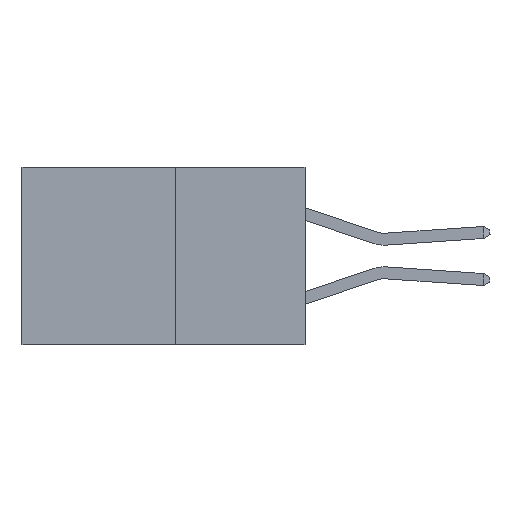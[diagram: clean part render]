
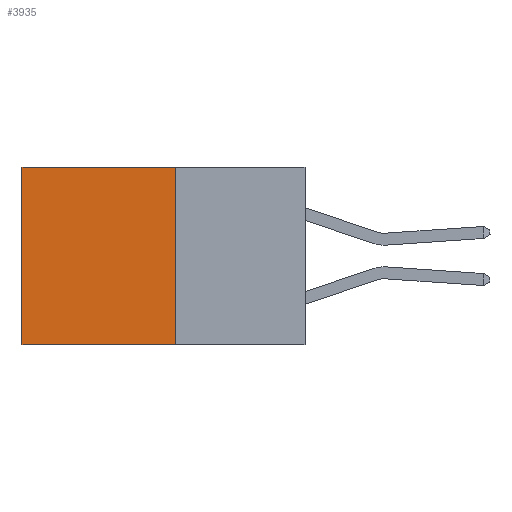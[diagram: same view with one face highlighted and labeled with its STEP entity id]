
A CAD part, left-side view. The second image highlights one B-rep face of the part: STEP entity #3935.
In plain terms, the highlighted planar face has unit normal (-1, 0, 0).
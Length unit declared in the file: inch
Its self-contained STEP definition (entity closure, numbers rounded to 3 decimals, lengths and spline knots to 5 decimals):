
#682 = LINE ( 'NONE', #12573, #7615 ) ;
#790 = CARTESIAN_POINT ( 'NONE',  ( 0.277, 0.59, -0.37 ) ) ;
#882 = CARTESIAN_POINT ( 'NONE',  ( 0.277, 0.59, -0.37 ) ) ;
#2208 = DIRECTION ( 'NONE',  ( 0., 0., -1. ) ) ;
#2367 = ORIENTED_EDGE ( 'NONE', *, *, #11489, .T. ) ;
#3160 = DIRECTION ( 'NONE',  ( 0., 0., -1. ) ) ;
#3935 = ADVANCED_FACE ( 'NONE', ( #9014 ), #6004, .F. ) ;
#4317 = DIRECTION ( 'NONE',  ( 0., 1., 0. ) ) ;
#4378 = AXIS2_PLACEMENT_3D ( 'NONE', #5776, #17102, #3160 ) ;
#5776 = CARTESIAN_POINT ( 'NONE',  ( 0.277, 0.27, -0.37 ) ) ;
#6004 = PLANE ( 'NONE',  #4378 ) ;
#6259 = VECTOR ( 'NONE', #2208, 39.37008 ) ;
#6675 = EDGE_CURVE ( 'NONE', #7914, #14545, #13708, .T. ) ;
#6972 = VERTEX_POINT ( 'NONE', #10802 ) ;
#7615 = VECTOR ( 'NONE', #12729, 39.37008 ) ;
#7914 = VERTEX_POINT ( 'NONE', #9151 ) ;
#8889 = EDGE_CURVE ( 'NONE', #7914, #6972, #682, .T. ) ;
#8963 = ORIENTED_EDGE ( 'NONE', *, *, #16537, .F. ) ;
#9014 = FACE_OUTER_BOUND ( 'NONE', #13960, .T. ) ;
#9151 = CARTESIAN_POINT ( 'NONE',  ( 0.277, 0.27, 0. ) ) ;
#9563 = VECTOR ( 'NONE', #4317, 39.37008 ) ;
#10131 = CARTESIAN_POINT ( 'NONE',  ( 0.277, 0.59, 0. ) ) ;
#10135 = VECTOR ( 'NONE', #12858, 39.37008 ) ;
#10167 = ORIENTED_EDGE ( 'NONE', *, *, #6675, .T. ) ;
#10802 = CARTESIAN_POINT ( 'NONE',  ( 0.277, 0.27, -0.37 ) ) ;
#10837 = LINE ( 'NONE', #790, #6259 ) ;
#11489 = EDGE_CURVE ( 'NONE', #14545, #16225, #10837, .T. ) ;
#11621 = ORIENTED_EDGE ( 'NONE', *, *, #8889, .F. ) ;
#12573 = CARTESIAN_POINT ( 'NONE',  ( 0.277, 0.27, -0.37 ) ) ;
#12729 = DIRECTION ( 'NONE',  ( 0., 0., -1. ) ) ;
#12858 = DIRECTION ( 'NONE',  ( 0., 1., 0. ) ) ;
#13189 = LINE ( 'NONE', #15194, #9563 ) ;
#13247 = CARTESIAN_POINT ( 'NONE',  ( 0.277, 0.27, 0. ) ) ;
#13708 = LINE ( 'NONE', #13247, #10135 ) ;
#13960 = EDGE_LOOP ( 'NONE', ( #2367, #8963, #11621, #10167 ) ) ;
#14545 = VERTEX_POINT ( 'NONE', #10131 ) ;
#15194 = CARTESIAN_POINT ( 'NONE',  ( 0.277, 0.27, -0.37 ) ) ;
#16225 = VERTEX_POINT ( 'NONE', #882 ) ;
#16537 = EDGE_CURVE ( 'NONE', #6972, #16225, #13189, .T. ) ;
#17102 = DIRECTION ( 'NONE',  ( 1., 0., 0. ) ) ;
